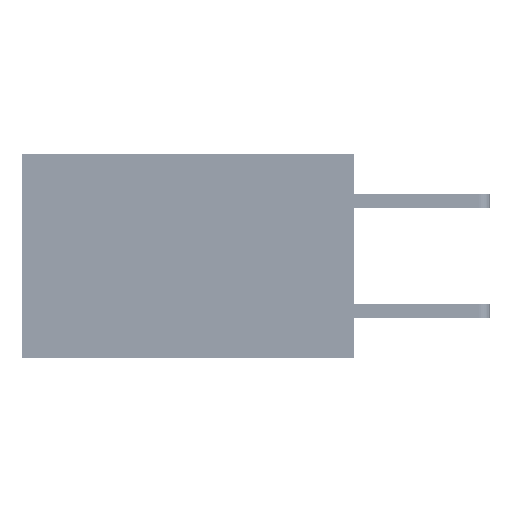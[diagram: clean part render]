
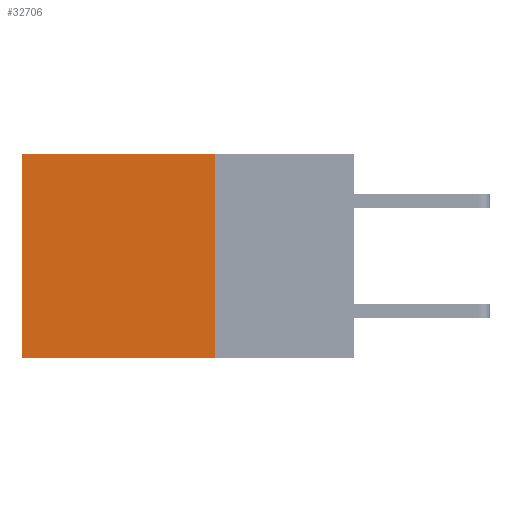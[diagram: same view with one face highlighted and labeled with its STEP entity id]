
A CAD part, left-side view. The second image highlights one B-rep face of the part: STEP entity #32706.
In plain terms, the highlighted planar face has unit normal (-1, 0, 0).
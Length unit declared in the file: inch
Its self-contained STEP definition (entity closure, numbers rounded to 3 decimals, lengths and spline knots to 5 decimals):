
#600 = VERTEX_POINT ( 'NONE', #48885 ) ;
#2061 = VERTEX_POINT ( 'NONE', #36389 ) ;
#2292 = AXIS2_PLACEMENT_3D ( 'NONE', #18083, #29900, #21358 ) ;
#3024 = FACE_OUTER_BOUND ( 'NONE', #21570, .T. ) ;
#3954 = VERTEX_POINT ( 'NONE', #7466 ) ;
#7466 = CARTESIAN_POINT ( 'NONE',  ( 0.2875, 0.25, -0.37 ) ) ;
#7688 = CARTESIAN_POINT ( 'NONE',  ( 0.2875, 0.6, 0. ) ) ;
#10701 = VECTOR ( 'NONE', #42624, 39.37008 ) ;
#12482 = CARTESIAN_POINT ( 'NONE',  ( 0.2875, 0.25, 0. ) ) ;
#13104 = VECTOR ( 'NONE', #33336, 39.37008 ) ;
#14068 = EDGE_CURVE ( 'NONE', #3954, #2061, #37704, .T. ) ;
#15316 = EDGE_CURVE ( 'NONE', #600, #38600, #25829, .T. ) ;
#15501 = EDGE_CURVE ( 'NONE', #600, #3954, #46138, .T. ) ;
#18083 = CARTESIAN_POINT ( 'NONE',  ( 0.2875, 0.25, 0. ) ) ;
#18260 = ORIENTED_EDGE ( 'NONE', *, *, #27915, .T. ) ;
#19099 = VECTOR ( 'NONE', #22992, 39.37008 ) ;
#19230 = CARTESIAN_POINT ( 'NONE',  ( 0.2875, 0.6, 0. ) ) ;
#21358 = DIRECTION ( 'NONE',  ( 0., 0., -1. ) ) ;
#21570 = EDGE_LOOP ( 'NONE', ( #18260, #34509, #36122, #31603 ) ) ;
#22992 = DIRECTION ( 'NONE',  ( 0., 0., -1. ) ) ;
#25829 = LINE ( 'NONE', #38095, #13104 ) ;
#27915 = EDGE_CURVE ( 'NONE', #38600, #2061, #34795, .T. ) ;
#29641 = PLANE ( 'NONE',  #2292 ) ;
#29900 = DIRECTION ( 'NONE',  ( 1., 0., 0. ) ) ;
#29939 = DIRECTION ( 'NONE',  ( 0., 1., 0. ) ) ;
#31603 = ORIENTED_EDGE ( 'NONE', *, *, #15316, .T. ) ;
#32706 = ADVANCED_FACE ( 'NONE', ( #3024 ), #29641, .F. ) ;
#33336 = DIRECTION ( 'NONE',  ( 0., 1., 0. ) ) ;
#34509 = ORIENTED_EDGE ( 'NONE', *, *, #14068, .F. ) ;
#34795 = LINE ( 'NONE', #7688, #19099 ) ;
#36122 = ORIENTED_EDGE ( 'NONE', *, *, #15501, .F. ) ;
#36389 = CARTESIAN_POINT ( 'NONE',  ( 0.2875, 0.6, -0.37 ) ) ;
#37704 = LINE ( 'NONE', #49272, #43602 ) ;
#38095 = CARTESIAN_POINT ( 'NONE',  ( 0.2875, 0.25, 0. ) ) ;
#38600 = VERTEX_POINT ( 'NONE', #19230 ) ;
#42624 = DIRECTION ( 'NONE',  ( 0., 0., -1. ) ) ;
#43602 = VECTOR ( 'NONE', #29939, 39.37008 ) ;
#46138 = LINE ( 'NONE', #12482, #10701 ) ;
#48885 = CARTESIAN_POINT ( 'NONE',  ( 0.2875, 0.25, 0. ) ) ;
#49272 = CARTESIAN_POINT ( 'NONE',  ( 0.2875, 0.25, -0.37 ) ) ;
